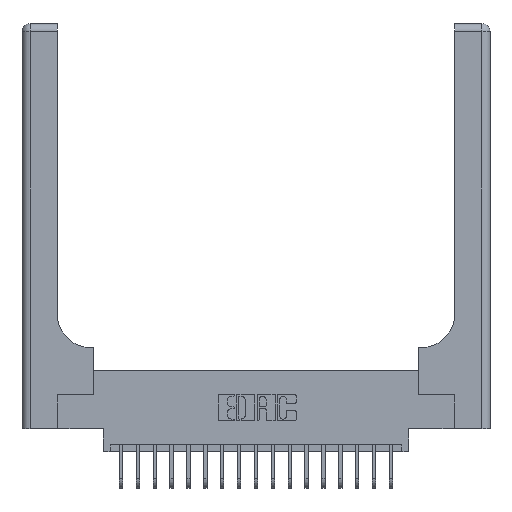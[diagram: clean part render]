
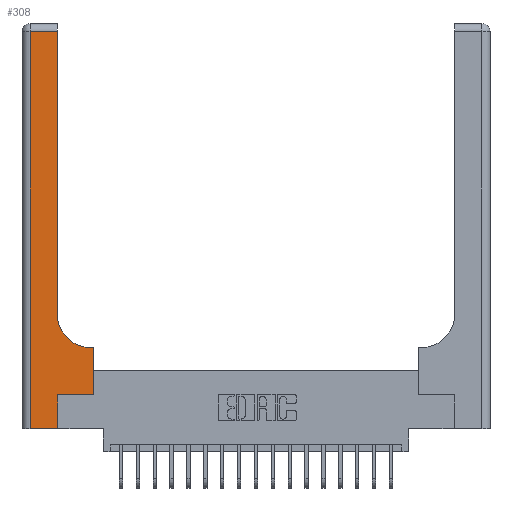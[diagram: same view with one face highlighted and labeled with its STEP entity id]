
A CAD part, top view. The second image highlights one B-rep face of the part: STEP entity #308.
In plain terms, the highlighted planar face has unit normal (0, 0, 1).
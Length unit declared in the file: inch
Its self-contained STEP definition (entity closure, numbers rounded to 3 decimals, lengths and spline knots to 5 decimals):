
#236 = LINE ( 'NONE', #15080, #15237 ) ;
#286 = EDGE_CURVE ( 'NONE', #6652, #19267, #6903, .T. ) ;
#308 = ADVANCED_FACE ( 'NONE', ( #2004 ), #12687, .F. ) ;
#752 = ORIENTED_EDGE ( 'NONE', *, *, #1773, .T. ) ;
#1006 = VECTOR ( 'NONE', #18604, 39.37008 ) ;
#1382 = CARTESIAN_POINT ( 'NONE',  ( 0.06, 0., 0.37 ) ) ;
#1773 = EDGE_CURVE ( 'NONE', #4032, #10106, #8955, .T. ) ;
#1930 = CARTESIAN_POINT ( 'NONE',  ( 0.528, 0.6, 0.37 ) ) ;
#2004 = FACE_OUTER_BOUND ( 'NONE', #3352, .T. ) ;
#2346 = EDGE_CURVE ( 'NONE', #10087, #7170, #15030, .T. ) ;
#2492 = DIRECTION ( 'NONE',  ( 1., 0., 0. ) ) ;
#3092 = VECTOR ( 'NONE', #10489, 39.37008 ) ;
#3352 = EDGE_LOOP ( 'NONE', ( #752, #13397, #3786, #8043, #8546, #18912, #16652, #7348, #5372 ) ) ;
#3449 = LINE ( 'NONE', #19257, #3912 ) ;
#3786 = ORIENTED_EDGE ( 'NONE', *, *, #286, .T. ) ;
#3912 = VECTOR ( 'NONE', #14834, 39.37008 ) ;
#4032 = VERTEX_POINT ( 'NONE', #13434 ) ;
#4234 = CARTESIAN_POINT ( 'NONE',  ( 0.528, 0.25, 0.37 ) ) ;
#4862 = CARTESIAN_POINT ( 'NONE',  ( 0., 2.94, 0.37 ) ) ;
#5372 = ORIENTED_EDGE ( 'NONE', *, *, #9062, .T. ) ;
#5486 = CARTESIAN_POINT ( 'NONE',  ( 0., 0., 0.37 ) ) ;
#5762 = VERTEX_POINT ( 'NONE', #18636 ) ;
#6152 = LINE ( 'NONE', #4862, #14128 ) ;
#6367 = DIRECTION ( 'NONE',  ( -1., 0., 0. ) ) ;
#6441 = VECTOR ( 'NONE', #13266, 39.37008 ) ;
#6652 = VERTEX_POINT ( 'NONE', #8823 ) ;
#6903 = LINE ( 'NONE', #13227, #6441 ) ;
#7058 = CARTESIAN_POINT ( 'NONE',  ( 0.51, 0.85, 0.37 ) ) ;
#7170 = VERTEX_POINT ( 'NONE', #4234 ) ;
#7181 = VECTOR ( 'NONE', #2492, 39.37008 ) ;
#7282 = LINE ( 'NONE', #8227, #11299 ) ;
#7348 = ORIENTED_EDGE ( 'NONE', *, *, #15072, .T. ) ;
#7589 = DIRECTION ( 'NONE',  ( -1., 0., 0. ) ) ;
#7888 = EDGE_CURVE ( 'NONE', #19267, #14081, #18625, .T. ) ;
#8043 = ORIENTED_EDGE ( 'NONE', *, *, #7888, .T. ) ;
#8124 = EDGE_CURVE ( 'NONE', #14081, #10087, #3449, .T. ) ;
#8227 = CARTESIAN_POINT ( 'NONE',  ( 0.528, 0.25, 0.37 ) ) ;
#8278 = AXIS2_PLACEMENT_3D ( 'NONE', #7058, #17525, #8581 ) ;
#8546 = ORIENTED_EDGE ( 'NONE', *, *, #8124, .T. ) ;
#8581 = DIRECTION ( 'NONE',  ( 1., 0., 0. ) ) ;
#8823 = CARTESIAN_POINT ( 'NONE',  ( 0.06, 2.94, 0.37 ) ) ;
#8955 = LINE ( 'NONE', #10523, #1006 ) ;
#9062 = EDGE_CURVE ( 'NONE', #5762, #4032, #16753, .T. ) ;
#10087 = VERTEX_POINT ( 'NONE', #15291 ) ;
#10106 = VERTEX_POINT ( 'NONE', #13785 ) ;
#10489 = DIRECTION ( 'NONE',  ( 1., 0., 0. ) ) ;
#10523 = CARTESIAN_POINT ( 'NONE',  ( 0.26, 3., 0.37 ) ) ;
#11299 = VECTOR ( 'NONE', #18654, 39.37008 ) ;
#11935 = CARTESIAN_POINT ( 'NONE',  ( 0.265, 0.25, 0.37 ) ) ;
#11972 = AXIS2_PLACEMENT_3D ( 'NONE', #12498, #12477, #12434 ) ;
#12434 = DIRECTION ( 'NONE',  ( -1., 0., 0. ) ) ;
#12477 = DIRECTION ( 'NONE',  ( 0., 0., -1. ) ) ;
#12498 = CARTESIAN_POINT ( 'NONE',  ( 0., 3., 0.37 ) ) ;
#12687 = PLANE ( 'NONE',  #11972 ) ;
#12693 = CARTESIAN_POINT ( 'NONE',  ( 0.265, 0., 0.37 ) ) ;
#13227 = CARTESIAN_POINT ( 'NONE',  ( 0.06, 3., 0.37 ) ) ;
#13266 = DIRECTION ( 'NONE',  ( 0., -1., 0. ) ) ;
#13397 = ORIENTED_EDGE ( 'NONE', *, *, #13450, .T. ) ;
#13434 = CARTESIAN_POINT ( 'NONE',  ( 0.26, 0.85, 0.37 ) ) ;
#13450 = EDGE_CURVE ( 'NONE', #10106, #6652, #6152, .T. ) ;
#13785 = CARTESIAN_POINT ( 'NONE',  ( 0.26, 2.94, 0.37 ) ) ;
#14081 = VERTEX_POINT ( 'NONE', #12693 ) ;
#14089 = EDGE_CURVE ( 'NONE', #7170, #18935, #7282, .T. ) ;
#14128 = VECTOR ( 'NONE', #6367, 39.37008 ) ;
#14834 = DIRECTION ( 'NONE',  ( 0., 1., 0. ) ) ;
#15030 = LINE ( 'NONE', #11935, #3092 ) ;
#15072 = EDGE_CURVE ( 'NONE', #18935, #5762, #236, .T. ) ;
#15080 = CARTESIAN_POINT ( 'NONE',  ( 0.26, 0.6, 0.37 ) ) ;
#15237 = VECTOR ( 'NONE', #7589, 39.37008 ) ;
#15291 = CARTESIAN_POINT ( 'NONE',  ( 0.265, 0.25, 0.37 ) ) ;
#16652 = ORIENTED_EDGE ( 'NONE', *, *, #14089, .T. ) ;
#16753 = CIRCLE ( 'NONE', #8278, 0.25 ) ;
#17525 = DIRECTION ( 'NONE',  ( 0., 0., -1. ) ) ;
#18604 = DIRECTION ( 'NONE',  ( 0., 1., 0. ) ) ;
#18625 = LINE ( 'NONE', #5486, #7181 ) ;
#18636 = CARTESIAN_POINT ( 'NONE',  ( 0.51, 0.6, 0.37 ) ) ;
#18654 = DIRECTION ( 'NONE',  ( 0., 1., 0. ) ) ;
#18912 = ORIENTED_EDGE ( 'NONE', *, *, #2346, .T. ) ;
#18935 = VERTEX_POINT ( 'NONE', #1930 ) ;
#19257 = CARTESIAN_POINT ( 'NONE',  ( 0.265, 0., 0.37 ) ) ;
#19267 = VERTEX_POINT ( 'NONE', #1382 ) ;
